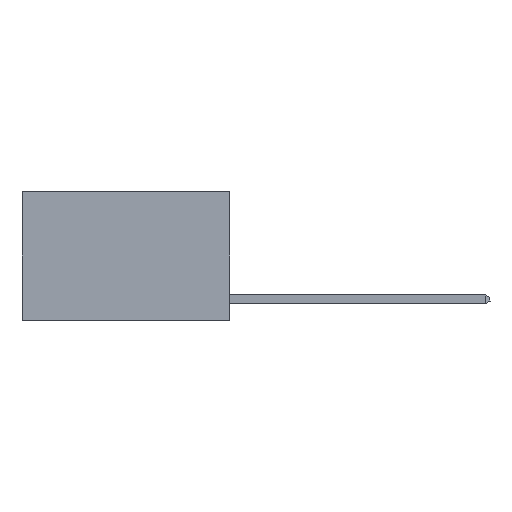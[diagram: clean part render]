
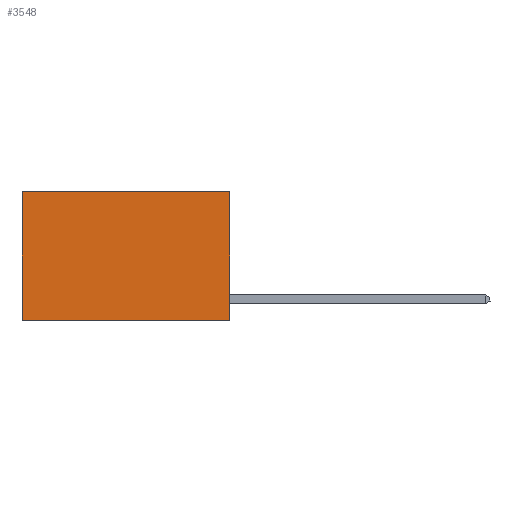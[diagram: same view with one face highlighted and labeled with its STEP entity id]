
A CAD part, left-side view. The second image highlights one B-rep face of the part: STEP entity #3548.
In plain terms, the highlighted planar face has unit normal (-1, 0, 0).
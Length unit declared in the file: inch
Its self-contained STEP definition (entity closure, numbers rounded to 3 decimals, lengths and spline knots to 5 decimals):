
#348 = ORIENTED_EDGE ( 'NONE', *, *, #12061, .F. ) ;
#367 = LINE ( 'NONE', #8191, #11163 ) ;
#576 = DIRECTION ( 'NONE',  ( 0., 0., -1. ) ) ;
#1066 = PLANE ( 'NONE',  #15443 ) ;
#1176 = LINE ( 'NONE', #4154, #8689 ) ;
#1478 = CARTESIAN_POINT ( 'NONE',  ( 0.2625, 0., 0. ) ) ;
#1647 = CARTESIAN_POINT ( 'NONE',  ( 0.2625, 0., -0.37 ) ) ;
#1877 = VERTEX_POINT ( 'NONE', #1478 ) ;
#2318 = EDGE_LOOP ( 'NONE', ( #12650, #348, #11443, #5554 ) ) ;
#2534 = VERTEX_POINT ( 'NONE', #8623 ) ;
#3488 = VERTEX_POINT ( 'NONE', #17647 ) ;
#3548 = ADVANCED_FACE ( 'NONE', ( #11579 ), #1066, .F. ) ;
#3564 = EDGE_CURVE ( 'NONE', #1877, #3856, #367, .T. ) ;
#3856 = VERTEX_POINT ( 'NONE', #1647 ) ;
#3870 = DIRECTION ( 'NONE',  ( 0., 0., -1. ) ) ;
#4154 = CARTESIAN_POINT ( 'NONE',  ( 0.2625, 0., 0. ) ) ;
#5554 = ORIENTED_EDGE ( 'NONE', *, *, #10623, .T. ) ;
#5652 = EDGE_CURVE ( 'NONE', #3488, #2534, #13530, .T. ) ;
#8191 = CARTESIAN_POINT ( 'NONE',  ( 0.2625, 0., 0. ) ) ;
#8623 = CARTESIAN_POINT ( 'NONE',  ( 0.2625, 0.6, -0.37 ) ) ;
#8689 = VECTOR ( 'NONE', #13987, 39.37008 ) ;
#9800 = VECTOR ( 'NONE', #576, 39.37008 ) ;
#10427 = CARTESIAN_POINT ( 'NONE',  ( 0.2625, 0.6, 0. ) ) ;
#10623 = EDGE_CURVE ( 'NONE', #1877, #3488, #1176, .T. ) ;
#10932 = CARTESIAN_POINT ( 'NONE',  ( 0.2625, 0., 0. ) ) ;
#11163 = VECTOR ( 'NONE', #15076, 39.37008 ) ;
#11443 = ORIENTED_EDGE ( 'NONE', *, *, #3564, .F. ) ;
#11579 = FACE_OUTER_BOUND ( 'NONE', #2318, .T. ) ;
#12061 = EDGE_CURVE ( 'NONE', #3856, #2534, #16868, .T. ) ;
#12324 = DIRECTION ( 'NONE',  ( 1., 0., 0. ) ) ;
#12650 = ORIENTED_EDGE ( 'NONE', *, *, #5652, .T. ) ;
#13530 = LINE ( 'NONE', #10427, #9800 ) ;
#13987 = DIRECTION ( 'NONE',  ( 0., 1., 0. ) ) ;
#14175 = DIRECTION ( 'NONE',  ( 0., 1., 0. ) ) ;
#15076 = DIRECTION ( 'NONE',  ( 0., 0., -1. ) ) ;
#15443 = AXIS2_PLACEMENT_3D ( 'NONE', #10932, #12324, #3870 ) ;
#15999 = VECTOR ( 'NONE', #14175, 39.37008 ) ;
#16868 = LINE ( 'NONE', #16934, #15999 ) ;
#16934 = CARTESIAN_POINT ( 'NONE',  ( 0.2625, 0., -0.37 ) ) ;
#17647 = CARTESIAN_POINT ( 'NONE',  ( 0.2625, 0.6, 0. ) ) ;
